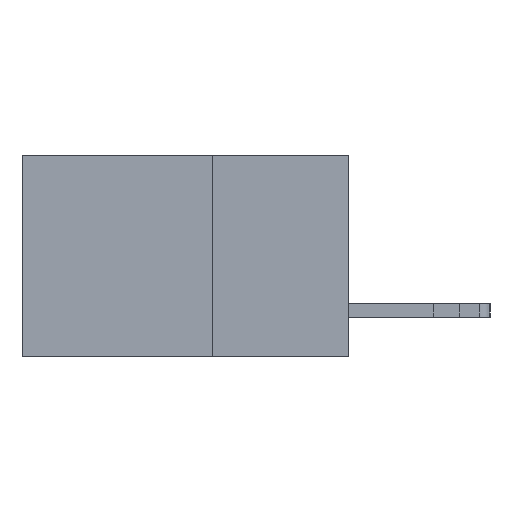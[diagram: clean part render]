
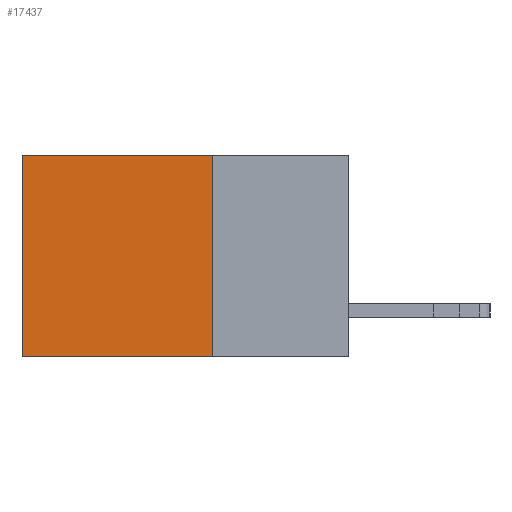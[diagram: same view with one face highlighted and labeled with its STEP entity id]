
A CAD part, left-side view. The second image highlights one B-rep face of the part: STEP entity #17437.
In plain terms, the highlighted planar face has unit normal (-1, 0, 0).
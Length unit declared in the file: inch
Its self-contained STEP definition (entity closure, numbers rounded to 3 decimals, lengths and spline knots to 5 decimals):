
#168 = EDGE_CURVE ( 'NONE', #3629, #12031, #6774, .T. ) ;
#2444 = CARTESIAN_POINT ( 'NONE',  ( 0.298, 0.25, 0. ) ) ;
#2751 = ORIENTED_EDGE ( 'NONE', *, *, #168, .T. ) ;
#2894 = CARTESIAN_POINT ( 'NONE',  ( 0.298, 0.6, -0.37 ) ) ;
#3629 = VERTEX_POINT ( 'NONE', #9893 ) ;
#4751 = VECTOR ( 'NONE', #19035, 39.37008 ) ;
#6228 = DIRECTION ( 'NONE',  ( 0., 1., 0. ) ) ;
#6354 = CARTESIAN_POINT ( 'NONE',  ( 0.298, 0.25, 0. ) ) ;
#6774 = LINE ( 'NONE', #10807, #11787 ) ;
#7491 = AXIS2_PLACEMENT_3D ( 'NONE', #13979, #7635, #22381 ) ;
#7635 = DIRECTION ( 'NONE',  ( 1., 0., 0. ) ) ;
#9709 = FACE_OUTER_BOUND ( 'NONE', #13167, .T. ) ;
#9893 = CARTESIAN_POINT ( 'NONE',  ( 0.298, 0.6, 0. ) ) ;
#10398 = CARTESIAN_POINT ( 'NONE',  ( 0.298, 0.25, -0.37 ) ) ;
#10542 = CARTESIAN_POINT ( 'NONE',  ( 0.298, 0.25, 0. ) ) ;
#10807 = CARTESIAN_POINT ( 'NONE',  ( 0.298, 0.6, 0. ) ) ;
#11659 = LINE ( 'NONE', #10398, #16645 ) ;
#11787 = VECTOR ( 'NONE', #23609, 39.37008 ) ;
#12031 = VERTEX_POINT ( 'NONE', #2894 ) ;
#13167 = EDGE_LOOP ( 'NONE', ( #2751, #26895, #26616, #25298 ) ) ;
#13979 = CARTESIAN_POINT ( 'NONE',  ( 0.298, 0.25, 0. ) ) ;
#14055 = LINE ( 'NONE', #10542, #23833 ) ;
#15380 = LINE ( 'NONE', #6354, #4751 ) ;
#16026 = VERTEX_POINT ( 'NONE', #22163 ) ;
#16645 = VECTOR ( 'NONE', #6228, 39.37008 ) ;
#17015 = EDGE_CURVE ( 'NONE', #21793, #16026, #15380, .T. ) ;
#17437 = ADVANCED_FACE ( 'NONE', ( #9709 ), #20284, .F. ) ;
#18168 = EDGE_CURVE ( 'NONE', #16026, #12031, #11659, .T. ) ;
#18949 = DIRECTION ( 'NONE',  ( 0., 1., 0. ) ) ;
#19035 = DIRECTION ( 'NONE',  ( 0., 0., -1. ) ) ;
#20284 = PLANE ( 'NONE',  #7491 ) ;
#21793 = VERTEX_POINT ( 'NONE', #2444 ) ;
#22163 = CARTESIAN_POINT ( 'NONE',  ( 0.298, 0.25, -0.37 ) ) ;
#22381 = DIRECTION ( 'NONE',  ( 0., 0., -1. ) ) ;
#23609 = DIRECTION ( 'NONE',  ( 0., 0., -1. ) ) ;
#23833 = VECTOR ( 'NONE', #18949, 39.37008 ) ;
#25298 = ORIENTED_EDGE ( 'NONE', *, *, #27344, .T. ) ;
#26616 = ORIENTED_EDGE ( 'NONE', *, *, #17015, .F. ) ;
#26895 = ORIENTED_EDGE ( 'NONE', *, *, #18168, .F. ) ;
#27344 = EDGE_CURVE ( 'NONE', #21793, #3629, #14055, .T. ) ;
